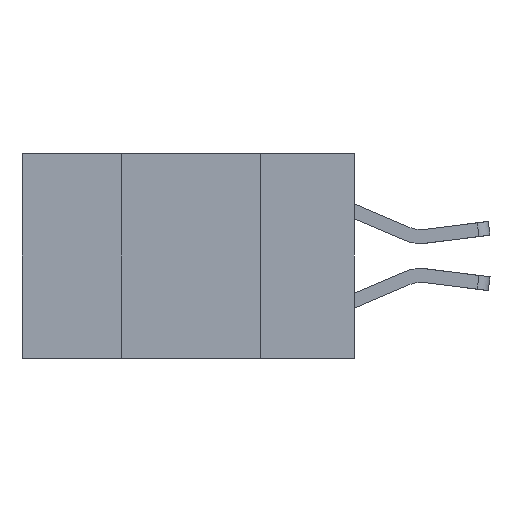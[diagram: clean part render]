
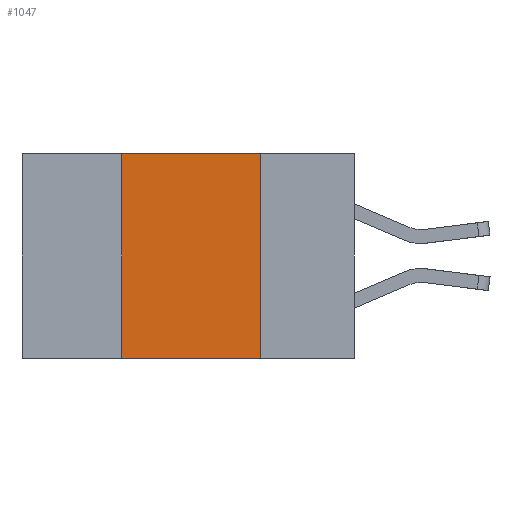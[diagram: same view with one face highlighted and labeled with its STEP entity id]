
A CAD part, left-side view. The second image highlights one B-rep face of the part: STEP entity #1047.
In plain terms, the highlighted planar face has unit normal (-1, 0, 0).
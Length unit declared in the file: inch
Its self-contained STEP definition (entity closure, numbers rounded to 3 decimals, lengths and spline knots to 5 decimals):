
#63 = PLANE ( 'NONE',  #5008 ) ;
#361 = DIRECTION ( 'NONE',  ( 0., 0., -1. ) ) ;
#397 = VERTEX_POINT ( 'NONE', #440 ) ;
#440 = CARTESIAN_POINT ( 'NONE',  ( 0., 0.17, -0.37 ) ) ;
#817 = EDGE_CURVE ( 'NONE', #832, #7339, #1774, .T. ) ;
#832 = VERTEX_POINT ( 'NONE', #8039 ) ;
#940 = VECTOR ( 'NONE', #8652, 39.37008 ) ;
#983 = ORIENTED_EDGE ( 'NONE', *, *, #1030, .T. ) ;
#993 = ORIENTED_EDGE ( 'NONE', *, *, #817, .F. ) ;
#1004 = ORIENTED_EDGE ( 'NONE', *, *, #1209, .F. ) ;
#1016 = ORIENTED_EDGE ( 'NONE', *, *, #1192, .F. ) ;
#1030 = EDGE_CURVE ( 'NONE', #832, #397, #3981, .T. ) ;
#1047 = ADVANCED_FACE ( 'NONE', ( #3743 ), #63, .F. ) ;
#1192 = EDGE_CURVE ( 'NONE', #2307, #397, #3362, .T. ) ;
#1209 = EDGE_CURVE ( 'NONE', #7339, #2307, #3116, .T. ) ;
#1774 = LINE ( 'NONE', #7141, #7077 ) ;
#2004 = CARTESIAN_POINT ( 'NONE',  ( 0., 0.17, 0. ) ) ;
#2307 = VERTEX_POINT ( 'NONE', #2004 ) ;
#3013 = EDGE_LOOP ( 'NONE', ( #1016, #1004, #993, #983 ) ) ;
#3116 = LINE ( 'NONE', #7796, #940 ) ;
#3362 = LINE ( 'NONE', #7555, #6673 ) ;
#3743 = FACE_OUTER_BOUND ( 'NONE', #3013, .T. ) ;
#3973 = DIRECTION ( 'NONE',  ( 0., 0., 1. ) ) ;
#3981 = LINE ( 'NONE', #8258, #8730 ) ;
#4694 = DIRECTION ( 'NONE',  ( 0., -1., 0. ) ) ;
#5008 = AXIS2_PLACEMENT_3D ( 'NONE', #8136, #8912, #361 ) ;
#6673 = VECTOR ( 'NONE', #7819, 39.37008 ) ;
#6915 = CARTESIAN_POINT ( 'NONE',  ( 0., 0.42, 0. ) ) ;
#7077 = VECTOR ( 'NONE', #3973, 39.37008 ) ;
#7141 = CARTESIAN_POINT ( 'NONE',  ( 0., 0.42, -0.37 ) ) ;
#7339 = VERTEX_POINT ( 'NONE', #6915 ) ;
#7555 = CARTESIAN_POINT ( 'NONE',  ( 0., 0.17, -0.37 ) ) ;
#7796 = CARTESIAN_POINT ( 'NONE',  ( 0., 0.6, 0. ) ) ;
#7819 = DIRECTION ( 'NONE',  ( 0., 0., -1. ) ) ;
#8039 = CARTESIAN_POINT ( 'NONE',  ( 0., 0.42, -0.37 ) ) ;
#8136 = CARTESIAN_POINT ( 'NONE',  ( 0., 0.6, 0. ) ) ;
#8258 = CARTESIAN_POINT ( 'NONE',  ( 0., 0.6, -0.37 ) ) ;
#8652 = DIRECTION ( 'NONE',  ( 0., -1., 0. ) ) ;
#8730 = VECTOR ( 'NONE', #4694, 39.37008 ) ;
#8912 = DIRECTION ( 'NONE',  ( 1., 0., 0. ) ) ;
